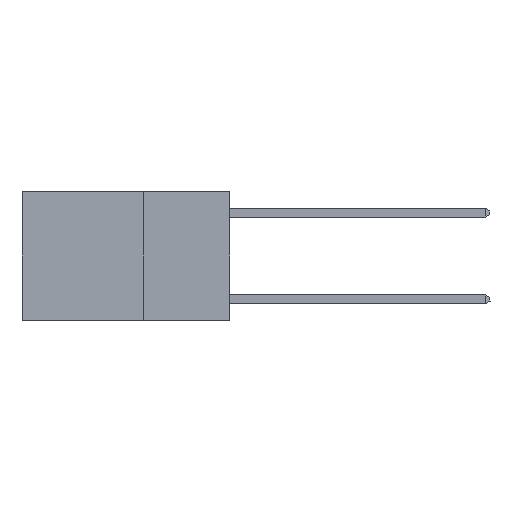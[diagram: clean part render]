
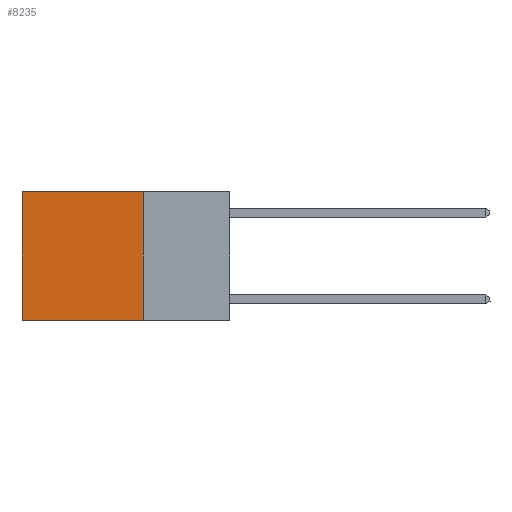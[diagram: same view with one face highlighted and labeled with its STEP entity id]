
A CAD part, left-side view. The second image highlights one B-rep face of the part: STEP entity #8235.
In plain terms, the highlighted planar face has unit normal (-1, 0, 0).
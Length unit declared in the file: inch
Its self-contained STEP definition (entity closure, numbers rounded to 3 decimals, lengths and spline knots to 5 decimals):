
#54 = LINE ( 'NONE', #8253, #3004 ) ;
#213 = FACE_OUTER_BOUND ( 'NONE', #6530, .T. ) ;
#549 = VECTOR ( 'NONE', #3046, 39.37008 ) ;
#986 = DIRECTION ( 'NONE',  ( 0., 1., 0. ) ) ;
#1224 = VERTEX_POINT ( 'NONE', #7764 ) ;
#1495 = ORIENTED_EDGE ( 'NONE', *, *, #15046, .T. ) ;
#1911 = CARTESIAN_POINT ( 'NONE',  ( 0.2625, 0.6, 0. ) ) ;
#2216 = VECTOR ( 'NONE', #15767, 39.37008 ) ;
#3004 = VECTOR ( 'NONE', #986, 39.37008 ) ;
#3015 = CARTESIAN_POINT ( 'NONE',  ( 0.2625, 0.25, -0.37 ) ) ;
#3046 = DIRECTION ( 'NONE',  ( 0., 0., -1. ) ) ;
#3211 = ORIENTED_EDGE ( 'NONE', *, *, #12618, .F. ) ;
#3242 = LINE ( 'NONE', #18450, #8296 ) ;
#3444 = AXIS2_PLACEMENT_3D ( 'NONE', #3713, #16654, #10846 ) ;
#3713 = CARTESIAN_POINT ( 'NONE',  ( 0.2625, 0.25, 0. ) ) ;
#5215 = DIRECTION ( 'NONE',  ( 0., 0., -1. ) ) ;
#5713 = EDGE_CURVE ( 'NONE', #17356, #6151, #6559, .T. ) ;
#6151 = VERTEX_POINT ( 'NONE', #11152 ) ;
#6530 = EDGE_LOOP ( 'NONE', ( #1495, #3211, #10017, #8563 ) ) ;
#6559 = LINE ( 'NONE', #12878, #2216 ) ;
#7764 = CARTESIAN_POINT ( 'NONE',  ( 0.2625, 0.6, -0.37 ) ) ;
#7858 = LINE ( 'NONE', #1911, #549 ) ;
#8235 = ADVANCED_FACE ( 'NONE', ( #213 ), #13663, .F. ) ;
#8253 = CARTESIAN_POINT ( 'NONE',  ( 0.2625, 0.25, -0.37 ) ) ;
#8296 = VECTOR ( 'NONE', #5215, 39.37008 ) ;
#8563 = ORIENTED_EDGE ( 'NONE', *, *, #5713, .T. ) ;
#10017 = ORIENTED_EDGE ( 'NONE', *, *, #15311, .F. ) ;
#10846 = DIRECTION ( 'NONE',  ( 0., 0., -1. ) ) ;
#11152 = CARTESIAN_POINT ( 'NONE',  ( 0.2625, 0.6, 0. ) ) ;
#11214 = VERTEX_POINT ( 'NONE', #3015 ) ;
#12618 = EDGE_CURVE ( 'NONE', #11214, #1224, #54, .T. ) ;
#12878 = CARTESIAN_POINT ( 'NONE',  ( 0.2625, 0.25, 0. ) ) ;
#13663 = PLANE ( 'NONE',  #3444 ) ;
#13888 = CARTESIAN_POINT ( 'NONE',  ( 0.2625, 0.25, 0. ) ) ;
#15046 = EDGE_CURVE ( 'NONE', #6151, #1224, #7858, .T. ) ;
#15311 = EDGE_CURVE ( 'NONE', #17356, #11214, #3242, .T. ) ;
#15767 = DIRECTION ( 'NONE',  ( 0., 1., 0. ) ) ;
#16654 = DIRECTION ( 'NONE',  ( 1., 0., 0. ) ) ;
#17356 = VERTEX_POINT ( 'NONE', #13888 ) ;
#18450 = CARTESIAN_POINT ( 'NONE',  ( 0.2625, 0.25, 0. ) ) ;
